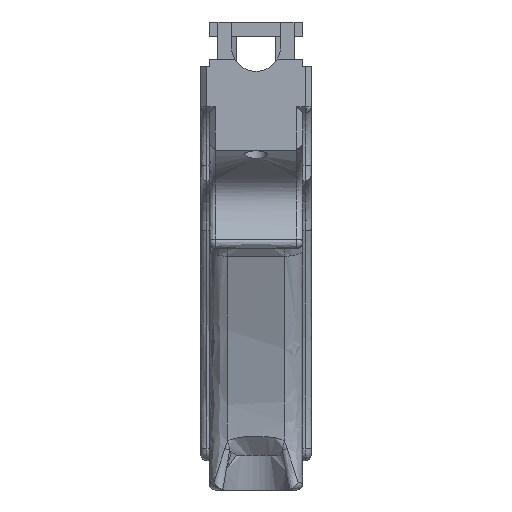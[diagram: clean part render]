
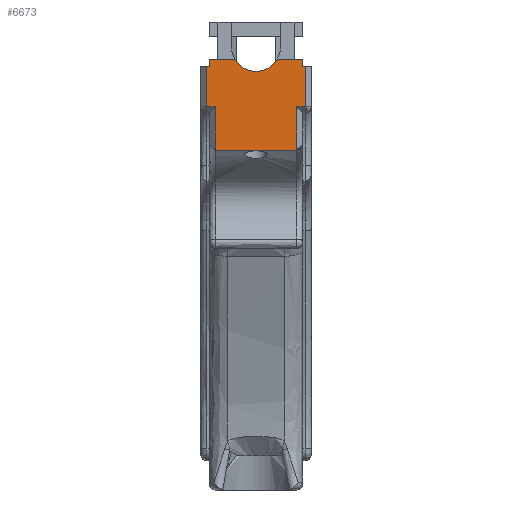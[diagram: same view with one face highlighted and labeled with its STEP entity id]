
A CAD part, front view. The second image highlights one B-rep face of the part: STEP entity #6673.
In plain terms, the highlighted planar face has unit normal (0, -1, 0).
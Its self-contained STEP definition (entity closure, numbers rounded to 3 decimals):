
#102=PLANE('',#7056);
#462=LINE('',#12579,#1094);
#467=LINE('',#12883,#1099);
#469=LINE('',#12887,#1101);
#470=LINE('',#12889,#1102);
#471=LINE('',#12891,#1103);
#472=LINE('',#12893,#1104);
#473=LINE('',#12895,#1105);
#474=LINE('',#12897,#1106);
#475=LINE('',#12899,#1107);
#476=LINE('',#12903,#1108);
#477=LINE('',#12905,#1109);
#478=LINE('',#12907,#1110);
#479=LINE('',#12909,#1111);
#480=LINE('',#12911,#1112);
#481=LINE('',#12912,#1113);
#1094=VECTOR('',#7811,10.);
#1099=VECTOR('',#7820,10.);
#1101=VECTOR('',#7824,10.);
#1102=VECTOR('',#7825,10.);
#1103=VECTOR('',#7826,10.);
#1104=VECTOR('',#7827,10.);
#1105=VECTOR('',#7828,10.);
#1106=VECTOR('',#7829,10.);
#1107=VECTOR('',#7830,10.);
#1108=VECTOR('',#7833,10.);
#1109=VECTOR('',#7834,10.);
#1110=VECTOR('',#7835,10.);
#1111=VECTOR('',#7836,10.);
#1112=VECTOR('',#7837,10.);
#1113=VECTOR('',#7838,10.);
#1759=FACE_OUTER_BOUND('',#2125,.T.);
#2125=EDGE_LOOP('',(#5063,#5064,#5065,#5066,#5067,#5068,#5069,#5070,#5071,
#5072,#5073,#5074,#5075,#5076,#5077,#5078));
#2445=CIRCLE('',#7057,4.2);
#2981=VERTEX_POINT('',#12576);
#2982=VERTEX_POINT('',#12578);
#2993=VERTEX_POINT('',#12882);
#2994=VERTEX_POINT('',#12886);
#2995=VERTEX_POINT('',#12888);
#2996=VERTEX_POINT('',#12890);
#2997=VERTEX_POINT('',#12892);
#2998=VERTEX_POINT('',#12894);
#2999=VERTEX_POINT('',#12896);
#3000=VERTEX_POINT('',#12898);
#3001=VERTEX_POINT('',#12900);
#3002=VERTEX_POINT('',#12902);
#3003=VERTEX_POINT('',#12904);
#3004=VERTEX_POINT('',#12906);
#3005=VERTEX_POINT('',#12908);
#3006=VERTEX_POINT('',#12910);
#3754=EDGE_CURVE('',#2982,#2981,#462,.T.);
#3770=EDGE_CURVE('',#2993,#2982,#467,.T.);
#3772=EDGE_CURVE('',#2994,#2981,#469,.F.);
#3773=EDGE_CURVE('',#2995,#2994,#470,.T.);
#3774=EDGE_CURVE('',#2996,#2995,#471,.T.);
#3775=EDGE_CURVE('',#2997,#2996,#472,.T.);
#3776=EDGE_CURVE('',#2997,#2998,#473,.T.);
#3777=EDGE_CURVE('',#2999,#2998,#474,.T.);
#3778=EDGE_CURVE('',#3000,#2999,#475,.T.);
#3779=EDGE_CURVE('',#3000,#3001,#2445,.T.);
#3780=EDGE_CURVE('',#3002,#3001,#476,.T.);
#3781=EDGE_CURVE('',#3003,#3002,#477,.T.);
#3782=EDGE_CURVE('',#3003,#3004,#478,.T.);
#3783=EDGE_CURVE('',#3005,#3004,#479,.T.);
#3784=EDGE_CURVE('',#3006,#3005,#480,.T.);
#3785=EDGE_CURVE('',#2993,#3006,#481,.T.);
#5063=ORIENTED_EDGE('',*,*,#3754,.T.);
#5064=ORIENTED_EDGE('',*,*,#3772,.F.);
#5065=ORIENTED_EDGE('',*,*,#3773,.F.);
#5066=ORIENTED_EDGE('',*,*,#3774,.F.);
#5067=ORIENTED_EDGE('',*,*,#3775,.F.);
#5068=ORIENTED_EDGE('',*,*,#3776,.T.);
#5069=ORIENTED_EDGE('',*,*,#3777,.F.);
#5070=ORIENTED_EDGE('',*,*,#3778,.F.);
#5071=ORIENTED_EDGE('',*,*,#3779,.T.);
#5072=ORIENTED_EDGE('',*,*,#3780,.F.);
#5073=ORIENTED_EDGE('',*,*,#3781,.F.);
#5074=ORIENTED_EDGE('',*,*,#3782,.T.);
#5075=ORIENTED_EDGE('',*,*,#3783,.F.);
#5076=ORIENTED_EDGE('',*,*,#3784,.F.);
#5077=ORIENTED_EDGE('',*,*,#3785,.F.);
#5078=ORIENTED_EDGE('',*,*,#3770,.T.);
#6673=ADVANCED_FACE('',(#1759),#102,.T.);
#7056=AXIS2_PLACEMENT_3D('',#12885,#7822,#7823);
#7057=AXIS2_PLACEMENT_3D('',#12901,#7831,#7832);
#7811=DIRECTION('',(1.,0.,0.));
#7820=DIRECTION('',(0.707,0.,-0.707));
#7822=DIRECTION('center_axis',(0.,-1.,0.));
#7823=DIRECTION('ref_axis',(0.,0.,-1.));
#7824=DIRECTION('',(0.707,0.,0.707));
#7825=DIRECTION('',(0.,0.,-1.));
#7826=DIRECTION('',(-1.,0.,0.));
#7827=DIRECTION('',(0.,0.,-1.));
#7828=DIRECTION('',(-1.,0.,0.));
#7829=DIRECTION('',(0.,0.,-1.));
#7830=DIRECTION('',(1.,0.,0.));
#7831=DIRECTION('center_axis',(0.,1.,0.));
#7832=DIRECTION('ref_axis',(1.,0.,0.));
#7833=DIRECTION('',(1.,0.,0.));
#7834=DIRECTION('',(0.,0.,1.));
#7835=DIRECTION('',(-1.,0.,0.));
#7836=DIRECTION('',(0.,0.,1.));
#7837=DIRECTION('',(-1.,0.,0.));
#7838=DIRECTION('',(0.,0.,1.));
#12576=CARTESIAN_POINT('',(14.843,-118.,-12.057));
#12578=CARTESIAN_POINT('',(1.057,-118.,-12.057));
#12579=CARTESIAN_POINT('',(3.974,-118.,-12.057));
#12882=CARTESIAN_POINT('',(1.,-118.,-12.));
#12883=CARTESIAN_POINT('',(-3.375,-118.,-7.625));
#12885=CARTESIAN_POINT('Origin',(0.,-118.,3.5));
#12886=CARTESIAN_POINT('',(14.9,-118.,-12.));
#12887=CARTESIAN_POINT('',(15.3,-118.,-11.6));
#12888=CARTESIAN_POINT('',(14.9,-118.,-4.6));
#12889=CARTESIAN_POINT('',(14.9,-118.,5.1));
#12890=CARTESIAN_POINT('',(16.4,-118.,-4.6));
#12891=CARTESIAN_POINT('',(0.725,-118.,-4.6));
#12892=CARTESIAN_POINT('',(16.4,-118.,2.25));
#12893=CARTESIAN_POINT('',(16.4,-118.,0.413));
#12894=CARTESIAN_POINT('',(15.9,-118.,2.25));
#12895=CARTESIAN_POINT('',(17.4,-118.,2.25));
#12896=CARTESIAN_POINT('',(15.9,-118.,3.5));
#12897=CARTESIAN_POINT('',(15.9,-118.,5.1));
#12898=CARTESIAN_POINT('',(11.544,-118.,3.5));
#12899=CARTESIAN_POINT('',(0.,-118.,3.5));
#12900=CARTESIAN_POINT('',(4.356,-118.,3.5));
#12901=CARTESIAN_POINT('Origin',(7.95,-118.,5.673));
#12902=CARTESIAN_POINT('',(0.,-118.,3.5));
#12903=CARTESIAN_POINT('',(0.,-118.,3.5));
#12904=CARTESIAN_POINT('',(0.,-118.,2.25));
#12905=CARTESIAN_POINT('',(0.,-118.,-7.95));
#12906=CARTESIAN_POINT('',(-0.5,-118.,2.25));
#12907=CARTESIAN_POINT('',(-1.5,-118.,2.25));
#12908=CARTESIAN_POINT('',(-0.5,-118.,-4.6));
#12909=CARTESIAN_POINT('',(-0.5,-118.,0.413));
#12910=CARTESIAN_POINT('',(1.,-118.,-4.6));
#12911=CARTESIAN_POINT('',(0.725,-118.,-4.6));
#12912=CARTESIAN_POINT('',(1.,-118.,-7.95));
